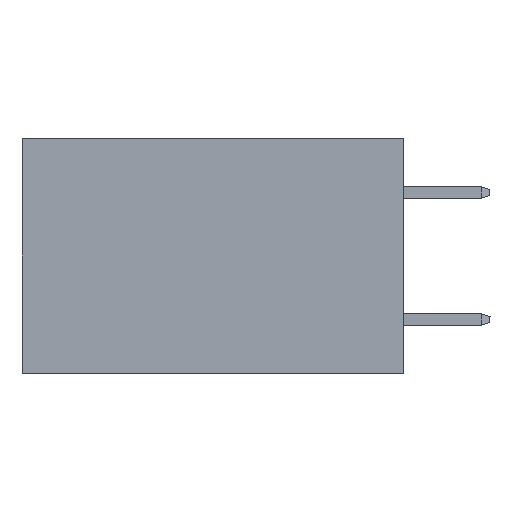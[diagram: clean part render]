
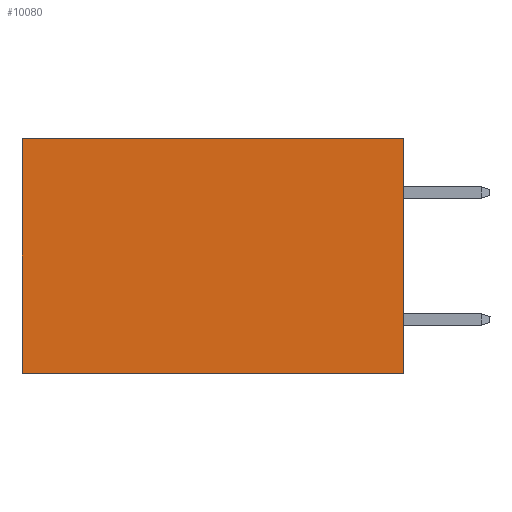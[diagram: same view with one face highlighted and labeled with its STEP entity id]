
A CAD part, left-side view. The second image highlights one B-rep face of the part: STEP entity #10080.
In plain terms, the highlighted planar face has unit normal (-1, 0, 0).
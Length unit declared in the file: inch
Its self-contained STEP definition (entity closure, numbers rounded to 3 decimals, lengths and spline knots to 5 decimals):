
#798 = VERTEX_POINT ( 'NONE', #6190 ) ;
#2107 = LINE ( 'NONE', #10228, #10715 ) ;
#2119 = PLANE ( 'NONE',  #9337 ) ;
#2630 = CARTESIAN_POINT ( 'NONE',  ( 0.2875, 0., 0. ) ) ;
#3541 = EDGE_LOOP ( 'NONE', ( #7960, #9920, #10503, #10878 ) ) ;
#3738 = LINE ( 'NONE', #2630, #13295 ) ;
#3939 = DIRECTION ( 'NONE',  ( 0., 0., -1. ) ) ;
#4730 = VERTEX_POINT ( 'NONE', #6077 ) ;
#5427 = DIRECTION ( 'NONE',  ( 0., 0., -1. ) ) ;
#5584 = FACE_OUTER_BOUND ( 'NONE', #3541, .T. ) ;
#5845 = CARTESIAN_POINT ( 'NONE',  ( 0.2875, 0., -0.37 ) ) ;
#5870 = LINE ( 'NONE', #14067, #10929 ) ;
#5942 = DIRECTION ( 'NONE',  ( 0., 1., 0. ) ) ;
#6077 = CARTESIAN_POINT ( 'NONE',  ( 0.2875, 0.6, -0.37 ) ) ;
#6145 = EDGE_CURVE ( 'NONE', #11955, #798, #10075, .T. ) ;
#6190 = CARTESIAN_POINT ( 'NONE',  ( 0.2875, 0.6, 0. ) ) ;
#6361 = VERTEX_POINT ( 'NONE', #5845 ) ;
#6617 = CARTESIAN_POINT ( 'NONE',  ( 0.2875, 0., 0. ) ) ;
#7592 = CARTESIAN_POINT ( 'NONE',  ( 0.2875, 0., 0. ) ) ;
#7779 = DIRECTION ( 'NONE',  ( 0., 1., 0. ) ) ;
#7960 = ORIENTED_EDGE ( 'NONE', *, *, #11234, .T. ) ;
#9337 = AXIS2_PLACEMENT_3D ( 'NONE', #6617, #13097, #3939 ) ;
#9630 = VECTOR ( 'NONE', #7779, 39.37008 ) ;
#9920 = ORIENTED_EDGE ( 'NONE', *, *, #12226, .F. ) ;
#10075 = LINE ( 'NONE', #13320, #9630 ) ;
#10080 = ADVANCED_FACE ( 'NONE', ( #5584 ), #2119, .F. ) ;
#10228 = CARTESIAN_POINT ( 'NONE',  ( 0.2875, 0.6, 0. ) ) ;
#10503 = ORIENTED_EDGE ( 'NONE', *, *, #12300, .F. ) ;
#10715 = VECTOR ( 'NONE', #5427, 39.37008 ) ;
#10878 = ORIENTED_EDGE ( 'NONE', *, *, #6145, .T. ) ;
#10929 = VECTOR ( 'NONE', #5942, 39.37008 ) ;
#11234 = EDGE_CURVE ( 'NONE', #798, #4730, #2107, .T. ) ;
#11955 = VERTEX_POINT ( 'NONE', #7592 ) ;
#12226 = EDGE_CURVE ( 'NONE', #6361, #4730, #5870, .T. ) ;
#12300 = EDGE_CURVE ( 'NONE', #11955, #6361, #3738, .T. ) ;
#12879 = DIRECTION ( 'NONE',  ( 0., 0., -1. ) ) ;
#13097 = DIRECTION ( 'NONE',  ( 1., 0., 0. ) ) ;
#13295 = VECTOR ( 'NONE', #12879, 39.37008 ) ;
#13320 = CARTESIAN_POINT ( 'NONE',  ( 0.2875, 0., 0. ) ) ;
#14067 = CARTESIAN_POINT ( 'NONE',  ( 0.2875, 0., -0.37 ) ) ;
